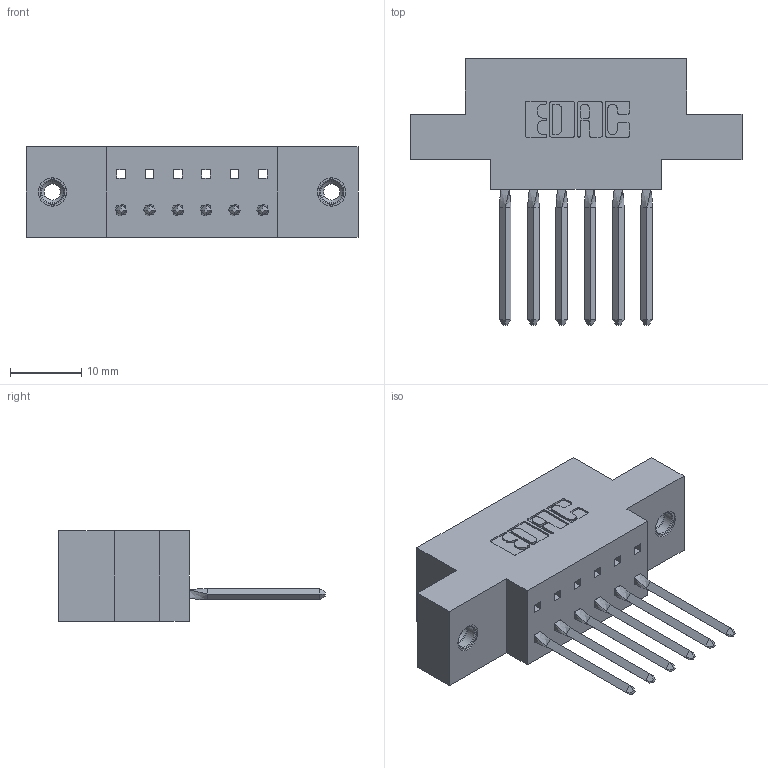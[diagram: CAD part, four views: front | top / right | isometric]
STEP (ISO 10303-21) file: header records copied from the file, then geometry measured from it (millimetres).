
FILE_DESCRIPTION (( 'STEP AP203' ), '1' );
FILE_NAME ('317-006-542-608.STEP', '2020-02-27T12:41:26', ( '' ), ( '' ), 'SwSTEP 2.0', 'SolidWorks 2016', '' );
FILE_SCHEMA (( 'CONFIG_CONTROL_DESIGN' ));
Length unit declared in the file: inch
Products named in the file (4): 345-250-001_345-250-003-102; 317 Part_.156 Dia - TI; 317-290-003_542; 317-006-542-608
Assembly tree (9 placements, depth 2):
  317-006-542-608
    317 Part_.156 Dia - TI
    317-290-003_542  x6
    345-250-001_345-250-003-102  x2
Bounding box: 46.48 x 37.34 x 12.7 mm (x, y, z)
Volume: 6216.5 mm3; surface area: 6799.8 mm2
Topology: 9 solids, 9 shells, 612 faces, 1713 edges, 1106 vertices
Faces by surface type: plane 474, cylinder 98, bspline 24, cone 12, torus 4
Entity records: 13706 total; most frequent: CARTESIAN_POINT 2634, ORIENTED_EDGE 2296, DIRECTION 2022, EDGE_CURVE 1148, LINE 958, VECTOR 958, VERTEX_POINT 756, AXIS2_PLACEMENT_3D 532
